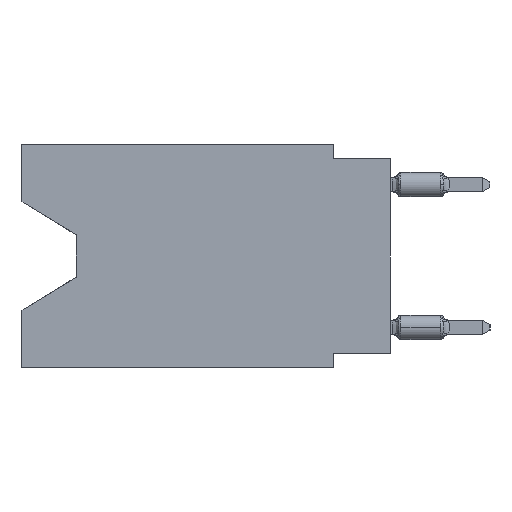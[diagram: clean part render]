
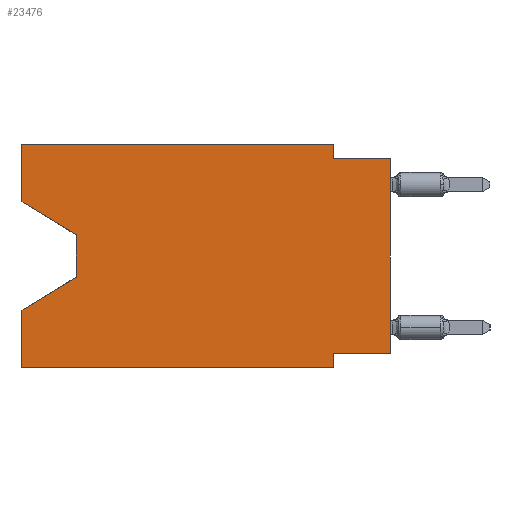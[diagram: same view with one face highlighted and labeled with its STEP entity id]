
A CAD part, left-side view. The second image highlights one B-rep face of the part: STEP entity #23476.
In plain terms, the highlighted planar face has unit normal (-1, 0, 0).
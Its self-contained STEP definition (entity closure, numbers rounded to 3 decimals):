
#341 = CARTESIAN_POINT ( 'NONE',  ( 0., 2.54, -9.906 ) ) ;
#360 = EDGE_LOOP ( 'NONE', ( #17031, #29576, #14210, #27934, #50745, #23381, #40827, #24762, #10490, #33266, #1736, #44281 ) ) ;
#447 = VECTOR ( 'NONE', #24779, 1000. ) ;
#1614 = VECTOR ( 'NONE', #45207, 1000. ) ;
#1736 = ORIENTED_EDGE ( 'NONE', *, *, #10870, .F. ) ;
#2479 = CARTESIAN_POINT ( 'NONE',  ( 0., 2.54, -9.906 ) ) ;
#2690 = CARTESIAN_POINT ( 'NONE',  ( 0., 16.383, -2.546 ) ) ;
#2844 = EDGE_CURVE ( 'NONE', #55532, #11534, #11398, .T. ) ;
#3867 = LINE ( 'NONE', #17989, #53934 ) ;
#4950 = LINE ( 'NONE', #14481, #28948 ) ;
#6313 = EDGE_CURVE ( 'NONE', #26456, #18831, #17285, .T. ) ;
#6426 = VERTEX_POINT ( 'NONE', #55924 ) ;
#8474 = DIRECTION ( 'NONE',  ( 0., 0., 1. ) ) ;
#9932 = CARTESIAN_POINT ( 'NONE',  ( 0., 16.383, 0. ) ) ;
#10457 = VERTEX_POINT ( 'NONE', #2479 ) ;
#10490 = ORIENTED_EDGE ( 'NONE', *, *, #51307, .F. ) ;
#10870 = EDGE_CURVE ( 'NONE', #17816, #26456, #31176, .T. ) ;
#11220 = CARTESIAN_POINT ( 'NONE',  ( 0., 0., -0.635 ) ) ;
#11342 = VERTEX_POINT ( 'NONE', #49803 ) ;
#11398 = LINE ( 'NONE', #29817, #33346 ) ;
#11534 = VERTEX_POINT ( 'NONE', #53117 ) ;
#11788 = CARTESIAN_POINT ( 'NONE',  ( 0., 0., 0. ) ) ;
#13610 = EDGE_CURVE ( 'NONE', #11342, #35932, #52677, .T. ) ;
#14170 = DIRECTION ( 'NONE',  ( 0., 0., -1. ) ) ;
#14210 = ORIENTED_EDGE ( 'NONE', *, *, #58259, .T. ) ;
#14481 = CARTESIAN_POINT ( 'NONE',  ( 0., 0., -0.635 ) ) ;
#14978 = CARTESIAN_POINT ( 'NONE',  ( 0., 13.97, -4.013 ) ) ;
#15200 = CARTESIAN_POINT ( 'NONE',  ( 0., 2.54, 0. ) ) ;
#15434 = CARTESIAN_POINT ( 'NONE',  ( 0., 16.383, -9.906 ) ) ;
#16822 = DIRECTION ( 'NONE',  ( 0., -1., 0. ) ) ;
#17031 = ORIENTED_EDGE ( 'NONE', *, *, #20622, .T. ) ;
#17285 = LINE ( 'NONE', #30798, #53066 ) ;
#17509 = VECTOR ( 'NONE', #16822, 1000. ) ;
#17816 = VERTEX_POINT ( 'NONE', #9932 ) ;
#17989 = CARTESIAN_POINT ( 'NONE',  ( 0., 13.97, -5.893 ) ) ;
#18286 = LINE ( 'NONE', #45297, #58033 ) ;
#18715 = DIRECTION ( 'NONE',  ( 1., 0., 0. ) ) ;
#18831 = VERTEX_POINT ( 'NONE', #43284 ) ;
#18837 = VECTOR ( 'NONE', #58060, 1000. ) ;
#19456 = EDGE_CURVE ( 'NONE', #40014, #10457, #21421, .T. ) ;
#20622 = EDGE_CURVE ( 'NONE', #6426, #11342, #49932, .T. ) ;
#20919 = DIRECTION ( 'NONE',  ( 0., 1., 0. ) ) ;
#21299 = VECTOR ( 'NONE', #14170, 1000. ) ;
#21421 = LINE ( 'NONE', #40132, #17509 ) ;
#21546 = CARTESIAN_POINT ( 'NONE',  ( 0., 16.383, -7.36 ) ) ;
#23381 = ORIENTED_EDGE ( 'NONE', *, *, #40291, .F. ) ;
#23476 = ADVANCED_FACE ( 'NONE', ( #56426 ), #55525, .F. ) ;
#24762 = ORIENTED_EDGE ( 'NONE', *, *, #37420, .T. ) ;
#24779 = DIRECTION ( 'NONE',  ( 0., 0., -1. ) ) ;
#25968 = DIRECTION ( 'NONE',  ( 0., -1., 0. ) ) ;
#26456 = VERTEX_POINT ( 'NONE', #15200 ) ;
#27203 = VERTEX_POINT ( 'NONE', #21546 ) ;
#27934 = ORIENTED_EDGE ( 'NONE', *, *, #32689, .F. ) ;
#28948 = VECTOR ( 'NONE', #50984, 1000. ) ;
#29006 = CARTESIAN_POINT ( 'NONE',  ( 0., 0., -9.271 ) ) ;
#29494 = VERTEX_POINT ( 'NONE', #11220 ) ;
#29576 = ORIENTED_EDGE ( 'NONE', *, *, #13610, .T. ) ;
#29817 = CARTESIAN_POINT ( 'NONE',  ( 0., 0., -9.271 ) ) ;
#30798 = CARTESIAN_POINT ( 'NONE',  ( 0., 2.54, 0. ) ) ;
#31176 = LINE ( 'NONE', #55088, #52246 ) ;
#32689 = EDGE_CURVE ( 'NONE', #40014, #27203, #39064, .T. ) ;
#33266 = ORIENTED_EDGE ( 'NONE', *, *, #6313, .F. ) ;
#33346 = VECTOR ( 'NONE', #20919, 1000. ) ;
#35932 = VERTEX_POINT ( 'NONE', #36090 ) ;
#36090 = CARTESIAN_POINT ( 'NONE',  ( 0., 13.97, -5.893 ) ) ;
#37420 = EDGE_CURVE ( 'NONE', #55532, #29494, #44598, .T. ) ;
#39064 = LINE ( 'NONE', #53454, #18837 ) ;
#40014 = VERTEX_POINT ( 'NONE', #15434 ) ;
#40132 = CARTESIAN_POINT ( 'NONE',  ( 0., 16.383, -9.906 ) ) ;
#40291 = EDGE_CURVE ( 'NONE', #11534, #10457, #42383, .T. ) ;
#40827 = ORIENTED_EDGE ( 'NONE', *, *, #2844, .F. ) ;
#42337 = DIRECTION ( 'NONE',  ( 0., 0., -1. ) ) ;
#42383 = LINE ( 'NONE', #341, #21299 ) ;
#42630 = CARTESIAN_POINT ( 'NONE',  ( 0., 16.383, 0. ) ) ;
#43284 = CARTESIAN_POINT ( 'NONE',  ( 0., 2.54, -0.635 ) ) ;
#44281 = ORIENTED_EDGE ( 'NONE', *, *, #46810, .F. ) ;
#44598 = LINE ( 'NONE', #11788, #1614 ) ;
#45207 = DIRECTION ( 'NONE',  ( 0., 0., 1. ) ) ;
#45297 = CARTESIAN_POINT ( 'NONE',  ( 0., 16.383, 0. ) ) ;
#45301 = DIRECTION ( 'NONE',  ( 0., 0.855, -0.519 ) ) ;
#45635 = DIRECTION ( 'NONE',  ( 0., -0.855, -0.519 ) ) ;
#46810 = EDGE_CURVE ( 'NONE', #6426, #17816, #18286, .T. ) ;
#49803 = CARTESIAN_POINT ( 'NONE',  ( 0., 13.97, -4.013 ) ) ;
#49932 = LINE ( 'NONE', #2690, #59739 ) ;
#50745 = ORIENTED_EDGE ( 'NONE', *, *, #19456, .T. ) ;
#50984 = DIRECTION ( 'NONE',  ( 0., -1., 0. ) ) ;
#51307 = EDGE_CURVE ( 'NONE', #18831, #29494, #4950, .T. ) ;
#52246 = VECTOR ( 'NONE', #25968, 1000. ) ;
#52677 = LINE ( 'NONE', #14978, #447 ) ;
#52680 = AXIS2_PLACEMENT_3D ( 'NONE', #42630, #18715, #42337 ) ;
#53066 = VECTOR ( 'NONE', #55011, 1000. ) ;
#53117 = CARTESIAN_POINT ( 'NONE',  ( 0., 2.54, -9.271 ) ) ;
#53454 = CARTESIAN_POINT ( 'NONE',  ( 0., 16.383, 0. ) ) ;
#53934 = VECTOR ( 'NONE', #45301, 1000. ) ;
#55011 = DIRECTION ( 'NONE',  ( 0., 0., -1. ) ) ;
#55088 = CARTESIAN_POINT ( 'NONE',  ( 0., 16.383, 0. ) ) ;
#55525 = PLANE ( 'NONE',  #52680 ) ;
#55532 = VERTEX_POINT ( 'NONE', #29006 ) ;
#55924 = CARTESIAN_POINT ( 'NONE',  ( 0., 16.383, -2.546 ) ) ;
#56426 = FACE_OUTER_BOUND ( 'NONE', #360, .T. ) ;
#58033 = VECTOR ( 'NONE', #8474, 1000. ) ;
#58060 = DIRECTION ( 'NONE',  ( 0., 0., 1. ) ) ;
#58259 = EDGE_CURVE ( 'NONE', #35932, #27203, #3867, .T. ) ;
#59739 = VECTOR ( 'NONE', #45635, 1000. ) ;
